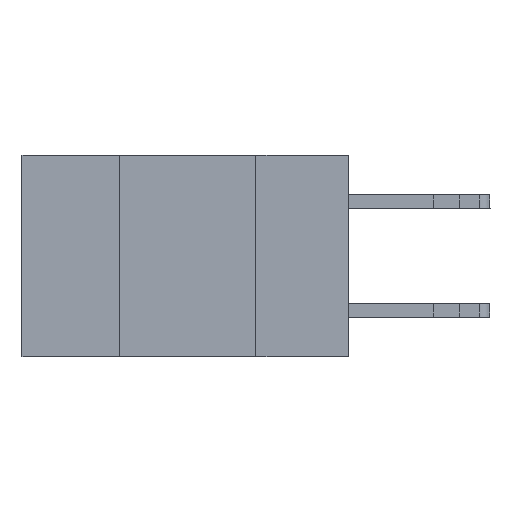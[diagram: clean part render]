
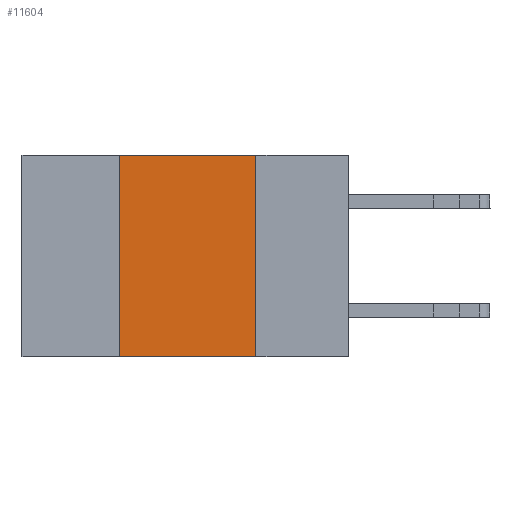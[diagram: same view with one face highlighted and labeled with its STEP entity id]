
A CAD part, left-side view. The second image highlights one B-rep face of the part: STEP entity #11604.
In plain terms, the highlighted planar face has unit normal (-1, 0, 0).
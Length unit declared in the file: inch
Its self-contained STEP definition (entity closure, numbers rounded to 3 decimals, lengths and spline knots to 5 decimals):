
#612 = VERTEX_POINT ( 'NONE', #9098 ) ;
#661 = ORIENTED_EDGE ( 'NONE', *, *, #6384, .F. ) ;
#721 = PLANE ( 'NONE',  #8513 ) ;
#851 = EDGE_CURVE ( 'NONE', #5031, #6732, #6656, .T. ) ;
#1732 = ORIENTED_EDGE ( 'NONE', *, *, #851, .F. ) ;
#1769 = VECTOR ( 'NONE', #9609, 39.37008 ) ;
#2666 = VERTEX_POINT ( 'NONE', #5472 ) ;
#2708 = DIRECTION ( 'NONE',  ( 1., 0., 0. ) ) ;
#3188 = CARTESIAN_POINT ( 'NONE',  ( 0., 0.17, -0.37 ) ) ;
#3653 = DIRECTION ( 'NONE',  ( 0., 0., -1. ) ) ;
#4078 = LINE ( 'NONE', #6706, #8897 ) ;
#4966 = DIRECTION ( 'NONE',  ( 0., -1., 0. ) ) ;
#5023 = DIRECTION ( 'NONE',  ( 0., 0., 1. ) ) ;
#5031 = VERTEX_POINT ( 'NONE', #5770 ) ;
#5428 = VECTOR ( 'NONE', #10290, 39.37008 ) ;
#5472 = CARTESIAN_POINT ( 'NONE',  ( 0., 0.42, -0.37 ) ) ;
#5681 = FACE_OUTER_BOUND ( 'NONE', #10896, .T. ) ;
#5770 = CARTESIAN_POINT ( 'NONE',  ( 0., 0.17, 0. ) ) ;
#6384 = EDGE_CURVE ( 'NONE', #2666, #612, #10706, .T. ) ;
#6593 = LINE ( 'NONE', #9412, #5428 ) ;
#6656 = LINE ( 'NONE', #10547, #1769 ) ;
#6706 = CARTESIAN_POINT ( 'NONE',  ( 0., 0.6, -0.37 ) ) ;
#6732 = VERTEX_POINT ( 'NONE', #3188 ) ;
#6761 = CARTESIAN_POINT ( 'NONE',  ( 0., 0.42, 0. ) ) ;
#6910 = ORIENTED_EDGE ( 'NONE', *, *, #7163, .T. ) ;
#7163 = EDGE_CURVE ( 'NONE', #2666, #6732, #4078, .T. ) ;
#8513 = AXIS2_PLACEMENT_3D ( 'NONE', #9286, #2708, #3653 ) ;
#8897 = VECTOR ( 'NONE', #4966, 39.37008 ) ;
#9098 = CARTESIAN_POINT ( 'NONE',  ( 0., 0.42, 0. ) ) ;
#9286 = CARTESIAN_POINT ( 'NONE',  ( 0., 0.6, 0. ) ) ;
#9412 = CARTESIAN_POINT ( 'NONE',  ( 0., 0.6, 0. ) ) ;
#9536 = EDGE_CURVE ( 'NONE', #612, #5031, #6593, .T. ) ;
#9609 = DIRECTION ( 'NONE',  ( 0., 0., -1. ) ) ;
#10290 = DIRECTION ( 'NONE',  ( 0., -1., 0. ) ) ;
#10547 = CARTESIAN_POINT ( 'NONE',  ( 0., 0.17, 0. ) ) ;
#10706 = LINE ( 'NONE', #6761, #10903 ) ;
#10896 = EDGE_LOOP ( 'NONE', ( #1732, #11297, #661, #6910 ) ) ;
#10903 = VECTOR ( 'NONE', #5023, 39.37008 ) ;
#11297 = ORIENTED_EDGE ( 'NONE', *, *, #9536, .F. ) ;
#11604 = ADVANCED_FACE ( 'NONE', ( #5681 ), #721, .F. ) ;
